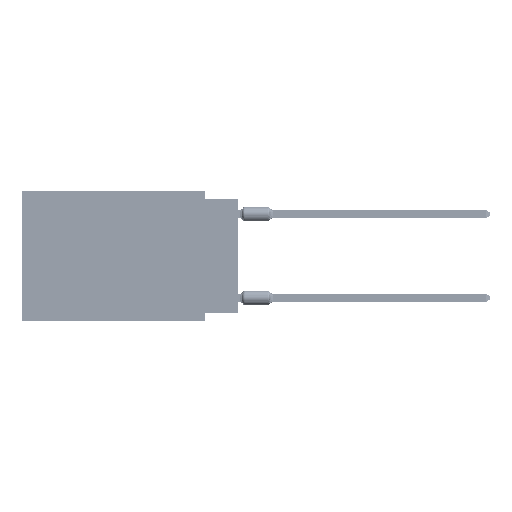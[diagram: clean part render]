
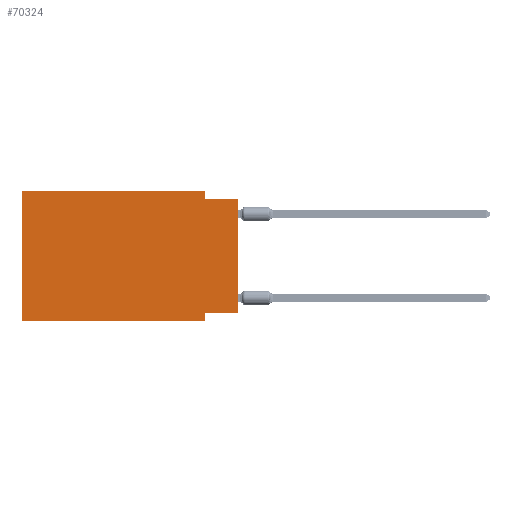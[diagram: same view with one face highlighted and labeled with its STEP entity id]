
A CAD part, left-side view. The second image highlights one B-rep face of the part: STEP entity #70324.
In plain terms, the highlighted planar face has unit normal (-1, 0, 0).
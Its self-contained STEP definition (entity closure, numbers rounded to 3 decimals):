
#992 = DIRECTION ( 'NONE',  ( 1., 0., 0. ) ) ;
#1591 = ORIENTED_EDGE ( 'NONE', *, *, #13585, .F. ) ;
#4763 = ORIENTED_EDGE ( 'NONE', *, *, #74346, .F. ) ;
#6503 = CARTESIAN_POINT ( 'NONE',  ( 0., 16.383, -9.906 ) ) ;
#7885 = CARTESIAN_POINT ( 'NONE',  ( 0., 16.383, 0. ) ) ;
#8424 = EDGE_CURVE ( 'NONE', #71422, #74956, #17418, .T. ) ;
#12869 = VERTEX_POINT ( 'NONE', #22716 ) ;
#13366 = VERTEX_POINT ( 'NONE', #61138 ) ;
#13585 = EDGE_CURVE ( 'NONE', #58941, #18568, #74530, .T. ) ;
#17418 = LINE ( 'NONE', #36085, #65782 ) ;
#17960 = ORIENTED_EDGE ( 'NONE', *, *, #44170, .F. ) ;
#18568 = VERTEX_POINT ( 'NONE', #75219 ) ;
#18969 = ORIENTED_EDGE ( 'NONE', *, *, #71257, .F. ) ;
#21266 = LINE ( 'NONE', #65095, #35940 ) ;
#21737 = ORIENTED_EDGE ( 'NONE', *, *, #26552, .T. ) ;
#22716 = CARTESIAN_POINT ( 'NONE',  ( 0., 0., -0.635 ) ) ;
#26552 = EDGE_CURVE ( 'NONE', #71422, #18568, #29679, .T. ) ;
#27873 = LINE ( 'NONE', #70916, #70808 ) ;
#28356 = VECTOR ( 'NONE', #55640, 1000. ) ;
#29679 = LINE ( 'NONE', #6503, #28356 ) ;
#32656 = DIRECTION ( 'NONE',  ( 0., 0., -1. ) ) ;
#32738 = VECTOR ( 'NONE', #36627, 1000. ) ;
#34696 = DIRECTION ( 'NONE',  ( 0., 0., -1. ) ) ;
#34761 = LINE ( 'NONE', #78604, #45168 ) ;
#35940 = VECTOR ( 'NONE', #46030, 1000. ) ;
#36085 = CARTESIAN_POINT ( 'NONE',  ( 0., 16.383, 0. ) ) ;
#36382 = CARTESIAN_POINT ( 'NONE',  ( 0., 0., -9.271 ) ) ;
#36475 = DIRECTION ( 'NONE',  ( 0., 0., 1. ) ) ;
#36497 = EDGE_CURVE ( 'NONE', #13366, #60199, #70049, .T. ) ;
#36627 = DIRECTION ( 'NONE',  ( 0., 1., 0. ) ) ;
#41361 = EDGE_CURVE ( 'NONE', #50508, #12869, #27873, .T. ) ;
#42321 = LINE ( 'NONE', #67087, #32738 ) ;
#44170 = EDGE_CURVE ( 'NONE', #60199, #12869, #21266, .T. ) ;
#44463 = VECTOR ( 'NONE', #34696, 1000. ) ;
#45168 = VECTOR ( 'NONE', #53053, 1000. ) ;
#46030 = DIRECTION ( 'NONE',  ( 0., -1., 0. ) ) ;
#50508 = VERTEX_POINT ( 'NONE', #36382 ) ;
#51590 = CARTESIAN_POINT ( 'NONE',  ( 0., 2.54, -0.635 ) ) ;
#52281 = CARTESIAN_POINT ( 'NONE',  ( 0., 2.54, -9.271 ) ) ;
#53053 = DIRECTION ( 'NONE',  ( 0., -1., 0. ) ) ;
#55640 = DIRECTION ( 'NONE',  ( 0., -1., 0. ) ) ;
#56620 = FACE_OUTER_BOUND ( 'NONE', #56836, .T. ) ;
#56660 = DIRECTION ( 'NONE',  ( 0., 0., -1. ) ) ;
#56836 = EDGE_LOOP ( 'NONE', ( #71386, #17960, #64008, #18969, #62664, #21737, #1591, #4763 ) ) ;
#58015 = CARTESIAN_POINT ( 'NONE',  ( 0., 16.383, 0. ) ) ;
#58941 = VERTEX_POINT ( 'NONE', #52281 ) ;
#59129 = DIRECTION ( 'NONE',  ( 0., 0., 1. ) ) ;
#60199 = VERTEX_POINT ( 'NONE', #51590 ) ;
#61138 = CARTESIAN_POINT ( 'NONE',  ( 0., 2.54, 0. ) ) ;
#62664 = ORIENTED_EDGE ( 'NONE', *, *, #8424, .F. ) ;
#63923 = PLANE ( 'NONE',  #78943 ) ;
#64008 = ORIENTED_EDGE ( 'NONE', *, *, #36497, .F. ) ;
#65095 = CARTESIAN_POINT ( 'NONE',  ( 0., 0., -0.635 ) ) ;
#65782 = VECTOR ( 'NONE', #36475, 1000. ) ;
#67087 = CARTESIAN_POINT ( 'NONE',  ( 0., 0., -9.271 ) ) ;
#69646 = CARTESIAN_POINT ( 'NONE',  ( 0., 2.54, -9.906 ) ) ;
#69972 = VECTOR ( 'NONE', #56660, 1000. ) ;
#70049 = LINE ( 'NONE', #70862, #44463 ) ;
#70324 = ADVANCED_FACE ( 'NONE', ( #56620 ), #63923, .F. ) ;
#70808 = VECTOR ( 'NONE', #59129, 1000. ) ;
#70862 = CARTESIAN_POINT ( 'NONE',  ( 0., 2.54, 0. ) ) ;
#70916 = CARTESIAN_POINT ( 'NONE',  ( 0., 0., 0. ) ) ;
#71257 = EDGE_CURVE ( 'NONE', #74956, #13366, #34761, .T. ) ;
#71386 = ORIENTED_EDGE ( 'NONE', *, *, #41361, .T. ) ;
#71422 = VERTEX_POINT ( 'NONE', #73708 ) ;
#73708 = CARTESIAN_POINT ( 'NONE',  ( 0., 16.383, -9.906 ) ) ;
#74346 = EDGE_CURVE ( 'NONE', #50508, #58941, #42321, .T. ) ;
#74530 = LINE ( 'NONE', #69646, #69972 ) ;
#74956 = VERTEX_POINT ( 'NONE', #58015 ) ;
#75219 = CARTESIAN_POINT ( 'NONE',  ( 0., 2.54, -9.906 ) ) ;
#78604 = CARTESIAN_POINT ( 'NONE',  ( 0., 16.383, 0. ) ) ;
#78943 = AXIS2_PLACEMENT_3D ( 'NONE', #7885, #992, #32656 ) ;
